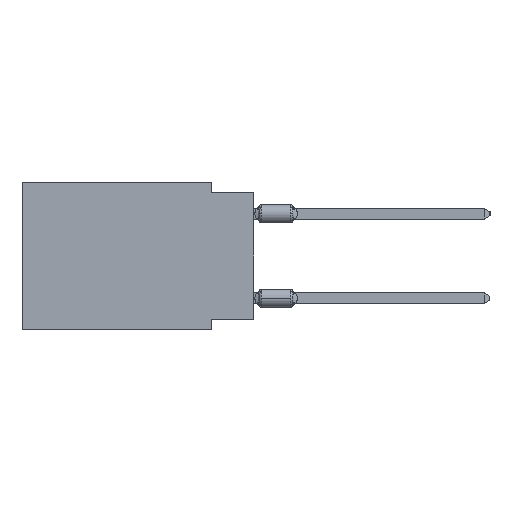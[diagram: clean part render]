
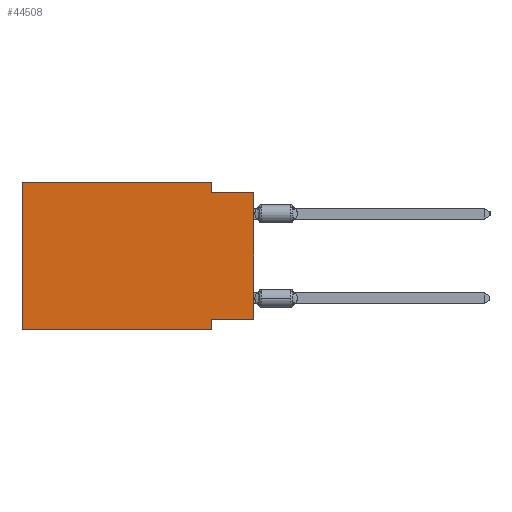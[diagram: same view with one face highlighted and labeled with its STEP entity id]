
A CAD part, left-side view. The second image highlights one B-rep face of the part: STEP entity #44508.
In plain terms, the highlighted planar face has unit normal (-1, 0, 0).
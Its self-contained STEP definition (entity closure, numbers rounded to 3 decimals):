
#481 = DIRECTION ( 'NONE',  ( 0., 0., -1. ) ) ;
#581 = LINE ( 'NONE', #20950, #16573 ) ;
#869 = DIRECTION ( 'NONE',  ( 0., 0., 1. ) ) ;
#1311 = LINE ( 'NONE', #45827, #27967 ) ;
#2337 = CARTESIAN_POINT ( 'NONE',  ( 0., 13.97, 0. ) ) ;
#3375 = CARTESIAN_POINT ( 'NONE',  ( 0., 2.54, 0. ) ) ;
#4444 = VERTEX_POINT ( 'NONE', #33235 ) ;
#5375 = CARTESIAN_POINT ( 'NONE',  ( 0., 2.54, -0.635 ) ) ;
#5828 = VERTEX_POINT ( 'NONE', #17182 ) ;
#7063 = DIRECTION ( 'NONE',  ( 0., 0., -1. ) ) ;
#7586 = DIRECTION ( 'NONE',  ( 0., 0., 1. ) ) ;
#7862 = VERTEX_POINT ( 'NONE', #3375 ) ;
#8257 = CARTESIAN_POINT ( 'NONE',  ( 0., 13.97, 0. ) ) ;
#9120 = DIRECTION ( 'NONE',  ( 0., -1., 0. ) ) ;
#12187 = ORIENTED_EDGE ( 'NONE', *, *, #25725, .F. ) ;
#12213 = DIRECTION ( 'NONE',  ( 0., -1., 0. ) ) ;
#13500 = ORIENTED_EDGE ( 'NONE', *, *, #23479, .F. ) ;
#13633 = ORIENTED_EDGE ( 'NONE', *, *, #41874, .F. ) ;
#14492 = CARTESIAN_POINT ( 'NONE',  ( 0., 13.97, -8.89 ) ) ;
#15013 = VECTOR ( 'NONE', #869, 1000. ) ;
#16573 = VECTOR ( 'NONE', #27322, 1000. ) ;
#16595 = VERTEX_POINT ( 'NONE', #5375 ) ;
#17182 = CARTESIAN_POINT ( 'NONE',  ( 0., 2.54, -8.255 ) ) ;
#18442 = FACE_OUTER_BOUND ( 'NONE', #32462, .T. ) ;
#20950 = CARTESIAN_POINT ( 'NONE',  ( 0., 0., -0.635 ) ) ;
#23193 = ORIENTED_EDGE ( 'NONE', *, *, #55759, .F. ) ;
#23479 = EDGE_CURVE ( 'NONE', #5828, #55731, #35222, .T. ) ;
#24352 = VECTOR ( 'NONE', #7586, 1000. ) ;
#25725 = EDGE_CURVE ( 'NONE', #16595, #26417, #581, .T. ) ;
#26417 = VERTEX_POINT ( 'NONE', #42794 ) ;
#27048 = ORIENTED_EDGE ( 'NONE', *, *, #66819, .F. ) ;
#27220 = VECTOR ( 'NONE', #12213, 1000. ) ;
#27322 = DIRECTION ( 'NONE',  ( 0., -1., 0. ) ) ;
#27804 = ORIENTED_EDGE ( 'NONE', *, *, #62486, .T. ) ;
#27947 = LINE ( 'NONE', #49632, #67904 ) ;
#27967 = VECTOR ( 'NONE', #44792, 1000. ) ;
#32200 = CARTESIAN_POINT ( 'NONE',  ( 0., 13.97, 0. ) ) ;
#32462 = EDGE_LOOP ( 'NONE', ( #27804, #12187, #51882, #27048, #23193, #45343, #13500, #13633 ) ) ;
#32864 = EDGE_CURVE ( 'NONE', #7862, #16595, #27947, .T. ) ;
#33235 = CARTESIAN_POINT ( 'NONE',  ( 0., 13.97, -8.89 ) ) ;
#34183 = CARTESIAN_POINT ( 'NONE',  ( 0., 2.54, -8.89 ) ) ;
#34843 = DIRECTION ( 'NONE',  ( 1., 0., 0. ) ) ;
#35222 = LINE ( 'NONE', #34183, #63130 ) ;
#35386 = LINE ( 'NONE', #8257, #27220 ) ;
#35960 = VERTEX_POINT ( 'NONE', #32200 ) ;
#37061 = VERTEX_POINT ( 'NONE', #46213 ) ;
#40164 = PLANE ( 'NONE',  #56788 ) ;
#41874 = EDGE_CURVE ( 'NONE', #37061, #5828, #1311, .T. ) ;
#42794 = CARTESIAN_POINT ( 'NONE',  ( 0., 0., -0.635 ) ) ;
#43662 = CARTESIAN_POINT ( 'NONE',  ( 0., 13.97, 0. ) ) ;
#44441 = VECTOR ( 'NONE', #9120, 1000. ) ;
#44508 = ADVANCED_FACE ( 'NONE', ( #18442 ), #40164, .F. ) ;
#44792 = DIRECTION ( 'NONE',  ( 0., 1., 0. ) ) ;
#45037 = LINE ( 'NONE', #50715, #24352 ) ;
#45343 = ORIENTED_EDGE ( 'NONE', *, *, #69192, .T. ) ;
#45827 = CARTESIAN_POINT ( 'NONE',  ( 0., 0., -8.255 ) ) ;
#45835 = DIRECTION ( 'NONE',  ( 0., 0., -1. ) ) ;
#46213 = CARTESIAN_POINT ( 'NONE',  ( 0., 0., -8.255 ) ) ;
#49632 = CARTESIAN_POINT ( 'NONE',  ( 0., 2.54, 0. ) ) ;
#50715 = CARTESIAN_POINT ( 'NONE',  ( 0., 0., 0. ) ) ;
#51882 = ORIENTED_EDGE ( 'NONE', *, *, #32864, .F. ) ;
#53988 = CARTESIAN_POINT ( 'NONE',  ( 0., 2.54, -8.89 ) ) ;
#54692 = LINE ( 'NONE', #43662, #15013 ) ;
#55731 = VERTEX_POINT ( 'NONE', #53988 ) ;
#55759 = EDGE_CURVE ( 'NONE', #4444, #35960, #54692, .T. ) ;
#56788 = AXIS2_PLACEMENT_3D ( 'NONE', #2337, #34843, #45835 ) ;
#62486 = EDGE_CURVE ( 'NONE', #37061, #26417, #45037, .T. ) ;
#63130 = VECTOR ( 'NONE', #7063, 1000. ) ;
#66819 = EDGE_CURVE ( 'NONE', #35960, #7862, #35386, .T. ) ;
#67904 = VECTOR ( 'NONE', #481, 1000. ) ;
#69192 = EDGE_CURVE ( 'NONE', #4444, #55731, #69714, .T. ) ;
#69714 = LINE ( 'NONE', #14492, #44441 ) ;
